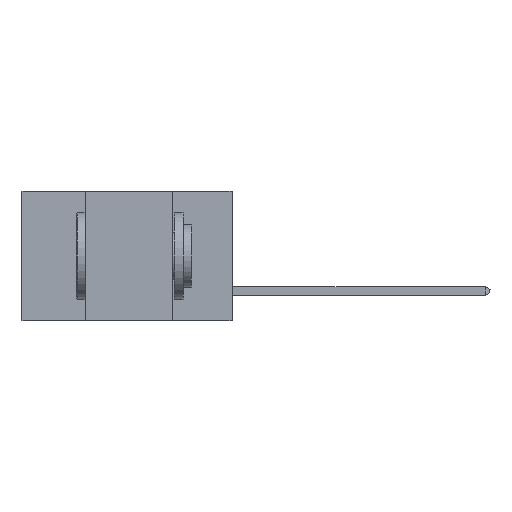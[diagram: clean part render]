
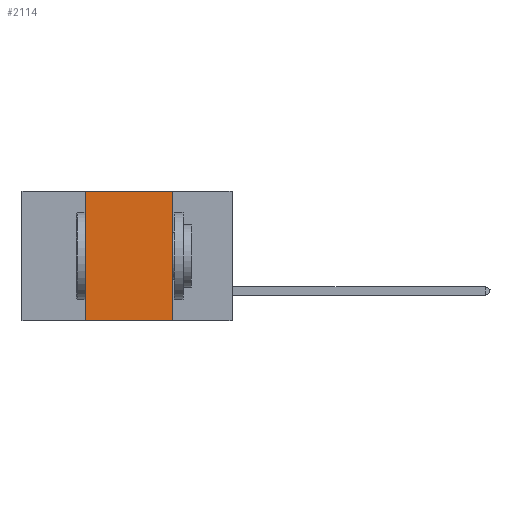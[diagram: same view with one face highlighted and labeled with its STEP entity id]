
A CAD part, left-side view. The second image highlights one B-rep face of the part: STEP entity #2114.
In plain terms, the highlighted planar face has unit normal (-1, 0, 0).
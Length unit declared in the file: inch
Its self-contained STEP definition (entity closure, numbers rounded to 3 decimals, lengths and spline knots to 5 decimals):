
#166 = CARTESIAN_POINT ( 'NONE',  ( 0., 0.42, -0.37 ) ) ;
#1952 = AXIS2_PLACEMENT_3D ( 'NONE', #14520, #16940, #25418 ) ;
#2114 = ADVANCED_FACE ( 'NONE', ( #2156 ), #14426, .F. ) ;
#2156 = FACE_OUTER_BOUND ( 'NONE', #8903, .T. ) ;
#3905 = DIRECTION ( 'NONE',  ( 0., -1., 0. ) ) ;
#3957 = EDGE_CURVE ( 'NONE', #26743, #16800, #16474, .T. ) ;
#4577 = EDGE_CURVE ( 'NONE', #26743, #19411, #16451, .T. ) ;
#7683 = ORIENTED_EDGE ( 'NONE', *, *, #3957, .T. ) ;
#8903 = EDGE_LOOP ( 'NONE', ( #10892, #22116, #25659, #7683 ) ) ;
#10892 = ORIENTED_EDGE ( 'NONE', *, *, #20514, .F. ) ;
#11392 = CARTESIAN_POINT ( 'NONE',  ( 0., 0.17, 0. ) ) ;
#11440 = DIRECTION ( 'NONE',  ( 0., 0., 1. ) ) ;
#12023 = VERTEX_POINT ( 'NONE', #21895 ) ;
#14011 = VECTOR ( 'NONE', #11440, 39.37008 ) ;
#14032 = VECTOR ( 'NONE', #15103, 39.37008 ) ;
#14426 = PLANE ( 'NONE',  #1952 ) ;
#14520 = CARTESIAN_POINT ( 'NONE',  ( 0., 0.6, 0. ) ) ;
#14793 = CARTESIAN_POINT ( 'NONE',  ( 0., 0.6, -0.37 ) ) ;
#15103 = DIRECTION ( 'NONE',  ( 0., -1., 0. ) ) ;
#16215 = LINE ( 'NONE', #11392, #16915 ) ;
#16451 = LINE ( 'NONE', #24827, #14011 ) ;
#16474 = LINE ( 'NONE', #14793, #23725 ) ;
#16800 = VERTEX_POINT ( 'NONE', #28267 ) ;
#16915 = VECTOR ( 'NONE', #22577, 39.37008 ) ;
#16940 = DIRECTION ( 'NONE',  ( 1., 0., 0. ) ) ;
#19411 = VERTEX_POINT ( 'NONE', #20816 ) ;
#20514 = EDGE_CURVE ( 'NONE', #12023, #16800, #16215, .T. ) ;
#20816 = CARTESIAN_POINT ( 'NONE',  ( 0., 0.42, 0. ) ) ;
#21895 = CARTESIAN_POINT ( 'NONE',  ( 0., 0.17, 0. ) ) ;
#22116 = ORIENTED_EDGE ( 'NONE', *, *, #22771, .F. ) ;
#22577 = DIRECTION ( 'NONE',  ( 0., 0., -1. ) ) ;
#22771 = EDGE_CURVE ( 'NONE', #19411, #12023, #26415, .T. ) ;
#23725 = VECTOR ( 'NONE', #3905, 39.37008 ) ;
#24827 = CARTESIAN_POINT ( 'NONE',  ( 0., 0.42, 0. ) ) ;
#25418 = DIRECTION ( 'NONE',  ( 0., 0., -1. ) ) ;
#25659 = ORIENTED_EDGE ( 'NONE', *, *, #4577, .F. ) ;
#26415 = LINE ( 'NONE', #28290, #14032 ) ;
#26743 = VERTEX_POINT ( 'NONE', #166 ) ;
#28267 = CARTESIAN_POINT ( 'NONE',  ( 0., 0.17, -0.37 ) ) ;
#28290 = CARTESIAN_POINT ( 'NONE',  ( 0., 0.6, 0. ) ) ;
